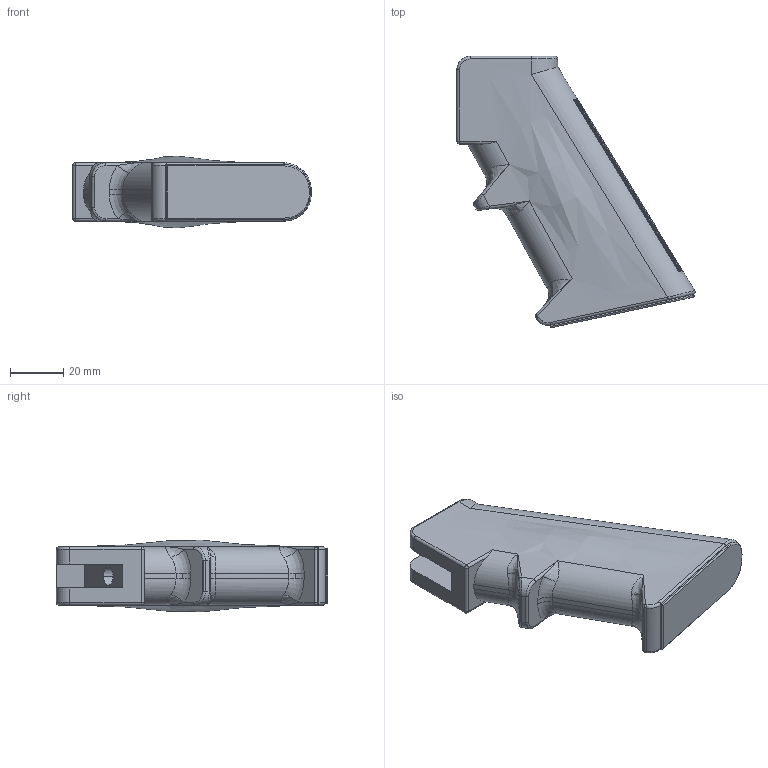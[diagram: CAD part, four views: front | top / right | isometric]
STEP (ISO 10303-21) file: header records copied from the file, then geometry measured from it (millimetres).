
FILE_DESCRIPTION (( 'STEP AP214' ), '1' );
FILE_NAME ('AR15GRIP.STEP', '2013-05-15T15:07:48', ( 'Asher' ), ( '' ), 'SwSTEP 2.0', 'SolidWorks 2013', '' );
FILE_SCHEMA (( 'AUTOMOTIVE_DESIGN' ));
Length unit declared in the file: inch
Products named in the file (1): AR15GRIP
Bounding box: 89.68 x 102.1 x 26.91 mm (x, y, z)
Volume: 60030.7 mm3; surface area: 26342.5 mm2
Topology: 1 solids, 1 shells, 171 faces, 397 edges, 232 vertices
Faces by surface type: cylinder 62, plane 61, bspline 37, torus 6, sphere 5
Entity records: 8841 total; most frequent: CARTESIAN_POINT 5495, ORIENTED_EDGE 778, DIRECTION 505, EDGE_CURVE 389, VERTEX_POINT 231, EDGE_LOOP 182, B_SPLINE_CURVE_WITH_KNOTS 172, AXIS2_PLACEMENT_3D 172
